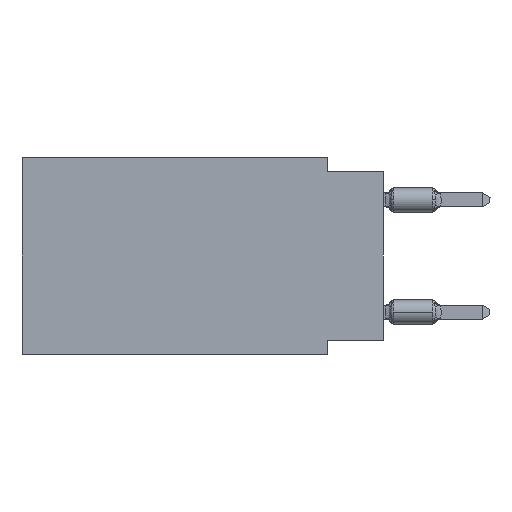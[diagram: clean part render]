
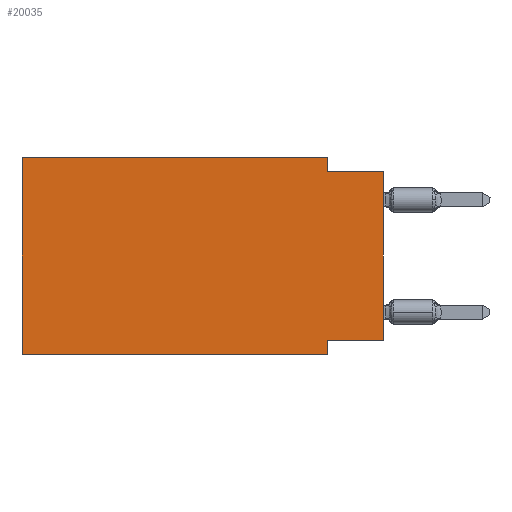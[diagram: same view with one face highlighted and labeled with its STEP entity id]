
A CAD part, left-side view. The second image highlights one B-rep face of the part: STEP entity #20035.
In plain terms, the highlighted planar face has unit normal (-1, 0, 0).
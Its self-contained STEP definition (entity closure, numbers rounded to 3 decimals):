
#1060 = CARTESIAN_POINT ( 'NONE',  ( 0., 2.54, -8.89 ) ) ;
#1520 = DIRECTION ( 'NONE',  ( 0., -1., 0. ) ) ;
#3480 = LINE ( 'NONE', #52863, #30061 ) ;
#4994 = ORIENTED_EDGE ( 'NONE', *, *, #50293, .T. ) ;
#5411 = CARTESIAN_POINT ( 'NONE',  ( 0., 16.383, 0. ) ) ;
#6851 = CARTESIAN_POINT ( 'NONE',  ( 0., 16.383, -8.89 ) ) ;
#9129 = VECTOR ( 'NONE', #1520, 1000. ) ;
#9220 = DIRECTION ( 'NONE',  ( 0., 0., -1. ) ) ;
#9642 = CARTESIAN_POINT ( 'NONE',  ( 0., 0., -8.255 ) ) ;
#9819 = EDGE_CURVE ( 'NONE', #15846, #55744, #12767, .T. ) ;
#12767 = LINE ( 'NONE', #51634, #60885 ) ;
#12970 = ORIENTED_EDGE ( 'NONE', *, *, #42862, .F. ) ;
#13284 = DIRECTION ( 'NONE',  ( 0., 0., 1. ) ) ;
#13710 = DIRECTION ( 'NONE',  ( 0., 0., 1. ) ) ;
#14131 = EDGE_CURVE ( 'NONE', #57510, #34350, #33881, .T. ) ;
#14142 = ORIENTED_EDGE ( 'NONE', *, *, #31067, .F. ) ;
#14671 = VERTEX_POINT ( 'NONE', #40688 ) ;
#14682 = DIRECTION ( 'NONE',  ( 1., 0., 0. ) ) ;
#15846 = VERTEX_POINT ( 'NONE', #56747 ) ;
#17422 = VECTOR ( 'NONE', #29097, 1000. ) ;
#17693 = ORIENTED_EDGE ( 'NONE', *, *, #9819, .F. ) ;
#20035 = ADVANCED_FACE ( 'NONE', ( #34105 ), #23592, .F. ) ;
#20076 = CARTESIAN_POINT ( 'NONE',  ( 0., 2.54, 0. ) ) ;
#23401 = LINE ( 'NONE', #47611, #29277 ) ;
#23592 = PLANE ( 'NONE',  #29754 ) ;
#25211 = EDGE_CURVE ( 'NONE', #62906, #49797, #3480, .T. ) ;
#25377 = VERTEX_POINT ( 'NONE', #53796 ) ;
#25768 = EDGE_CURVE ( 'NONE', #15846, #25377, #36831, .T. ) ;
#27356 = EDGE_LOOP ( 'NONE', ( #4994, #29904, #41210, #14142, #17693, #51173, #12970, #55429 ) ) ;
#28047 = VECTOR ( 'NONE', #50194, 1000. ) ;
#29097 = DIRECTION ( 'NONE',  ( 0., 1., 0. ) ) ;
#29277 = VECTOR ( 'NONE', #37125, 1000. ) ;
#29754 = AXIS2_PLACEMENT_3D ( 'NONE', #38241, #14682, #43647 ) ;
#29780 = LINE ( 'NONE', #1060, #33343 ) ;
#29904 = ORIENTED_EDGE ( 'NONE', *, *, #48003, .F. ) ;
#30061 = VECTOR ( 'NONE', #9220, 1000. ) ;
#31067 = EDGE_CURVE ( 'NONE', #55744, #62906, #56004, .T. ) ;
#33343 = VECTOR ( 'NONE', #44719, 1000. ) ;
#33881 = LINE ( 'NONE', #9642, #17422 ) ;
#34105 = FACE_OUTER_BOUND ( 'NONE', #27356, .T. ) ;
#34350 = VERTEX_POINT ( 'NONE', #53485 ) ;
#36831 = LINE ( 'NONE', #6851, #28047 ) ;
#37125 = DIRECTION ( 'NONE',  ( 0., -1., 0. ) ) ;
#38241 = CARTESIAN_POINT ( 'NONE',  ( 0., 16.383, 0. ) ) ;
#40688 = CARTESIAN_POINT ( 'NONE',  ( 0., 0., -0.635 ) ) ;
#41210 = ORIENTED_EDGE ( 'NONE', *, *, #25211, .F. ) ;
#42862 = EDGE_CURVE ( 'NONE', #34350, #25377, #29780, .T. ) ;
#43254 = CARTESIAN_POINT ( 'NONE',  ( 0., 2.54, -0.635 ) ) ;
#43647 = DIRECTION ( 'NONE',  ( 0., 0., -1. ) ) ;
#44719 = DIRECTION ( 'NONE',  ( 0., 0., -1. ) ) ;
#45178 = CARTESIAN_POINT ( 'NONE',  ( 0., 16.383, 0. ) ) ;
#47611 = CARTESIAN_POINT ( 'NONE',  ( 0., 0., -0.635 ) ) ;
#48003 = EDGE_CURVE ( 'NONE', #49797, #14671, #23401, .T. ) ;
#49797 = VERTEX_POINT ( 'NONE', #43254 ) ;
#50194 = DIRECTION ( 'NONE',  ( 0., -1., 0. ) ) ;
#50293 = EDGE_CURVE ( 'NONE', #57510, #14671, #55436, .T. ) ;
#51173 = ORIENTED_EDGE ( 'NONE', *, *, #25768, .T. ) ;
#51634 = CARTESIAN_POINT ( 'NONE',  ( 0., 16.383, 0. ) ) ;
#52863 = CARTESIAN_POINT ( 'NONE',  ( 0., 2.54, 0. ) ) ;
#53485 = CARTESIAN_POINT ( 'NONE',  ( 0., 2.54, -8.255 ) ) ;
#53796 = CARTESIAN_POINT ( 'NONE',  ( 0., 2.54, -8.89 ) ) ;
#55429 = ORIENTED_EDGE ( 'NONE', *, *, #14131, .F. ) ;
#55436 = LINE ( 'NONE', #55742, #59946 ) ;
#55742 = CARTESIAN_POINT ( 'NONE',  ( 0., 0., 0. ) ) ;
#55744 = VERTEX_POINT ( 'NONE', #5411 ) ;
#56004 = LINE ( 'NONE', #45178, #9129 ) ;
#56747 = CARTESIAN_POINT ( 'NONE',  ( 0., 16.383, -8.89 ) ) ;
#57510 = VERTEX_POINT ( 'NONE', #60137 ) ;
#59946 = VECTOR ( 'NONE', #13284, 1000. ) ;
#60137 = CARTESIAN_POINT ( 'NONE',  ( 0., 0., -8.255 ) ) ;
#60885 = VECTOR ( 'NONE', #13710, 1000. ) ;
#62906 = VERTEX_POINT ( 'NONE', #20076 ) ;
